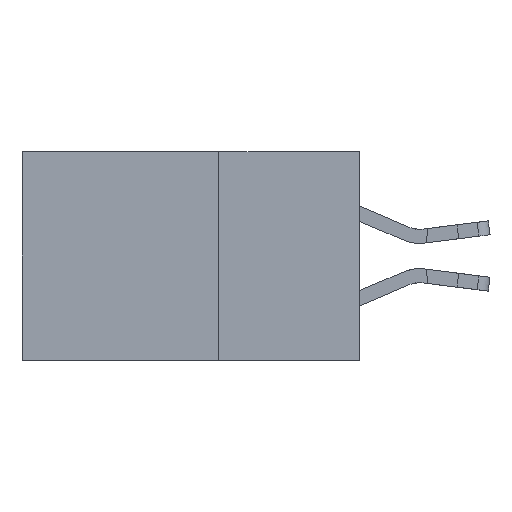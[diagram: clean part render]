
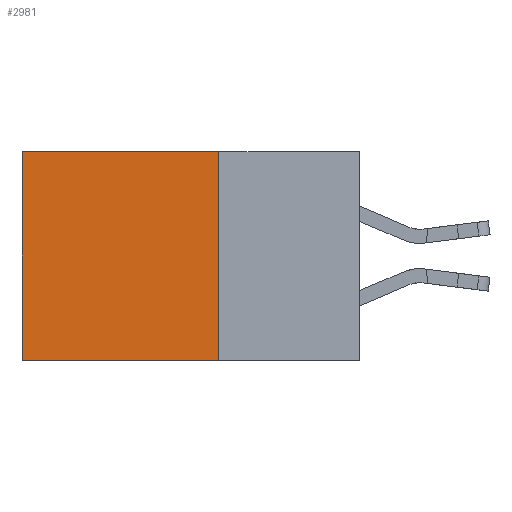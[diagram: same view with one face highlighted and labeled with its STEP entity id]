
A CAD part, left-side view. The second image highlights one B-rep face of the part: STEP entity #2981.
In plain terms, the highlighted planar face has unit normal (-1, 0, 0).
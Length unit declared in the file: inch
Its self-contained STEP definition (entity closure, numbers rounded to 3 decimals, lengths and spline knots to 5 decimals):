
#910 = FACE_OUTER_BOUND ( 'NONE', #13305, .T. ) ;
#1468 = AXIS2_PLACEMENT_3D ( 'NONE', #6336, #16500, #3402 ) ;
#2981 = ADVANCED_FACE ( 'NONE', ( #910 ), #18023, .F. ) ;
#3096 = DIRECTION ( 'NONE',  ( 0., 1., 0. ) ) ;
#3402 = DIRECTION ( 'NONE',  ( 0., 0., -1. ) ) ;
#3636 = CARTESIAN_POINT ( 'NONE',  ( 0.2875, 0.25, -0.37 ) ) ;
#3815 = LINE ( 'NONE', #5245, #11384 ) ;
#4672 = EDGE_CURVE ( 'NONE', #14465, #15963, #7268, .T. ) ;
#5085 = DIRECTION ( 'NONE',  ( 0., 1., 0. ) ) ;
#5193 = VERTEX_POINT ( 'NONE', #3636 ) ;
#5245 = CARTESIAN_POINT ( 'NONE',  ( 0.2875, 0.25, 0. ) ) ;
#5316 = ORIENTED_EDGE ( 'NONE', *, *, #6025, .T. ) ;
#5819 = CARTESIAN_POINT ( 'NONE',  ( 0.2875, 0.25, 0. ) ) ;
#6025 = EDGE_CURVE ( 'NONE', #15963, #8532, #8694, .T. ) ;
#6336 = CARTESIAN_POINT ( 'NONE',  ( 0.2875, 0.25, 0. ) ) ;
#6728 = CARTESIAN_POINT ( 'NONE',  ( 0.2875, 0.6, -0.37 ) ) ;
#6980 = DIRECTION ( 'NONE',  ( 0., 0., -1. ) ) ;
#7268 = LINE ( 'NONE', #12001, #8577 ) ;
#7579 = ORIENTED_EDGE ( 'NONE', *, *, #16031, .F. ) ;
#7697 = VECTOR ( 'NONE', #5085, 39.37008 ) ;
#8011 = LINE ( 'NONE', #9717, #7697 ) ;
#8532 = VERTEX_POINT ( 'NONE', #6728 ) ;
#8577 = VECTOR ( 'NONE', #3096, 39.37008 ) ;
#8694 = LINE ( 'NONE', #14179, #10408 ) ;
#9717 = CARTESIAN_POINT ( 'NONE',  ( 0.2875, 0.25, -0.37 ) ) ;
#10408 = VECTOR ( 'NONE', #6980, 39.37008 ) ;
#11384 = VECTOR ( 'NONE', #18246, 39.37008 ) ;
#11609 = ORIENTED_EDGE ( 'NONE', *, *, #17911, .F. ) ;
#12001 = CARTESIAN_POINT ( 'NONE',  ( 0.2875, 0.25, 0. ) ) ;
#13304 = ORIENTED_EDGE ( 'NONE', *, *, #4672, .T. ) ;
#13305 = EDGE_LOOP ( 'NONE', ( #5316, #7579, #11609, #13304 ) ) ;
#14179 = CARTESIAN_POINT ( 'NONE',  ( 0.2875, 0.6, 0. ) ) ;
#14465 = VERTEX_POINT ( 'NONE', #5819 ) ;
#14954 = CARTESIAN_POINT ( 'NONE',  ( 0.2875, 0.6, 0. ) ) ;
#15963 = VERTEX_POINT ( 'NONE', #14954 ) ;
#16031 = EDGE_CURVE ( 'NONE', #5193, #8532, #8011, .T. ) ;
#16500 = DIRECTION ( 'NONE',  ( 1., 0., 0. ) ) ;
#17911 = EDGE_CURVE ( 'NONE', #14465, #5193, #3815, .T. ) ;
#18023 = PLANE ( 'NONE',  #1468 ) ;
#18246 = DIRECTION ( 'NONE',  ( 0., 0., -1. ) ) ;
